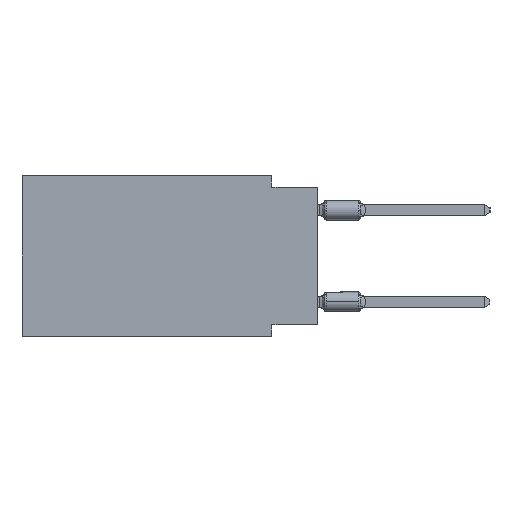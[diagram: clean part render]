
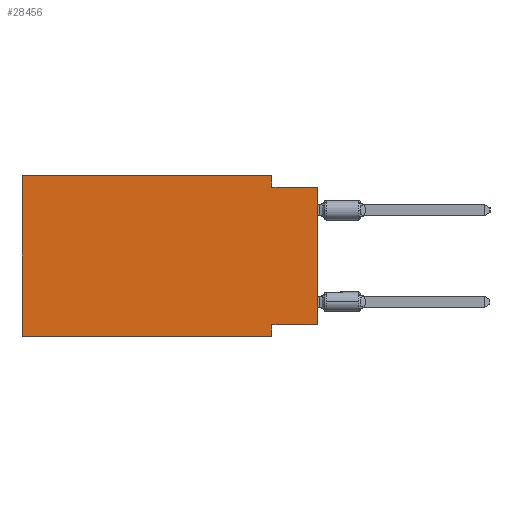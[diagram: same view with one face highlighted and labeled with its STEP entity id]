
A CAD part, left-side view. The second image highlights one B-rep face of the part: STEP entity #28456.
In plain terms, the highlighted planar face has unit normal (-1, 0, 0).
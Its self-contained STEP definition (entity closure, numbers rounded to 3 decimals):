
#618 = EDGE_CURVE ( 'NONE', #53708, #17051, #42193, .T. ) ;
#4104 = CARTESIAN_POINT ( 'NONE',  ( 0., 16.383, 0. ) ) ;
#4220 = ORIENTED_EDGE ( 'NONE', *, *, #20151, .F. ) ;
#5010 = VECTOR ( 'NONE', #34080, 1000. ) ;
#5094 = PLANE ( 'NONE',  #58560 ) ;
#6887 = CARTESIAN_POINT ( 'NONE',  ( 0., 0., -0.635 ) ) ;
#7912 = VECTOR ( 'NONE', #18733, 1000. ) ;
#11517 = CARTESIAN_POINT ( 'NONE',  ( 0., 0., 0. ) ) ;
#12225 = LINE ( 'NONE', #44247, #46390 ) ;
#13264 = EDGE_CURVE ( 'NONE', #17971, #17051, #45311, .T. ) ;
#13983 = ORIENTED_EDGE ( 'NONE', *, *, #56285, .F. ) ;
#17051 = VERTEX_POINT ( 'NONE', #6887 ) ;
#17971 = VERTEX_POINT ( 'NONE', #45802 ) ;
#18733 = DIRECTION ( 'NONE',  ( 0., -1., 0. ) ) ;
#19631 = VECTOR ( 'NONE', #56861, 1000. ) ;
#19765 = CARTESIAN_POINT ( 'NONE',  ( 0., 16.383, 0. ) ) ;
#20151 = EDGE_CURVE ( 'NONE', #31543, #17971, #60841, .T. ) ;
#21318 = EDGE_CURVE ( 'NONE', #53708, #58305, #46108, .T. ) ;
#24702 = ORIENTED_EDGE ( 'NONE', *, *, #34564, .T. ) ;
#24918 = CARTESIAN_POINT ( 'NONE',  ( 0., 0., -8.255 ) ) ;
#25700 = EDGE_CURVE ( 'NONE', #61450, #31543, #46005, .T. ) ;
#26708 = ORIENTED_EDGE ( 'NONE', *, *, #21318, .F. ) ;
#28456 = ADVANCED_FACE ( 'NONE', ( #51433 ), #5094, .F. ) ;
#30171 = DIRECTION ( 'NONE',  ( 0., 0., -1. ) ) ;
#31422 = CARTESIAN_POINT ( 'NONE',  ( 0., 2.54, 0. ) ) ;
#31543 = VERTEX_POINT ( 'NONE', #31422 ) ;
#33011 = DIRECTION ( 'NONE',  ( 0., 0., -1. ) ) ;
#33421 = ORIENTED_EDGE ( 'NONE', *, *, #25700, .F. ) ;
#33478 = CARTESIAN_POINT ( 'NONE',  ( 0., 16.383, 0. ) ) ;
#34080 = DIRECTION ( 'NONE',  ( 0., -1., 0. ) ) ;
#34564 = EDGE_CURVE ( 'NONE', #39815, #61401, #39172, .T. ) ;
#35756 = DIRECTION ( 'NONE',  ( 1., 0., 0. ) ) ;
#36201 = DIRECTION ( 'NONE',  ( 0., 1., 0. ) ) ;
#36923 = VECTOR ( 'NONE', #36201, 1000. ) ;
#38734 = ORIENTED_EDGE ( 'NONE', *, *, #618, .T. ) ;
#39172 = LINE ( 'NONE', #59972, #5010 ) ;
#39815 = VERTEX_POINT ( 'NONE', #63737 ) ;
#39867 = CARTESIAN_POINT ( 'NONE',  ( 0., 2.54, -8.89 ) ) ;
#41205 = DIRECTION ( 'NONE',  ( 0., 0., -1. ) ) ;
#42193 = LINE ( 'NONE', #11517, #19631 ) ;
#42225 = VECTOR ( 'NONE', #30171, 1000. ) ;
#42566 = ORIENTED_EDGE ( 'NONE', *, *, #13264, .F. ) ;
#44247 = CARTESIAN_POINT ( 'NONE',  ( 0., 2.54, -8.89 ) ) ;
#44613 = VECTOR ( 'NONE', #49166, 1000. ) ;
#44979 = DIRECTION ( 'NONE',  ( 0., -1., 0. ) ) ;
#45311 = LINE ( 'NONE', #45990, #7912 ) ;
#45802 = CARTESIAN_POINT ( 'NONE',  ( 0., 2.54, -0.635 ) ) ;
#45990 = CARTESIAN_POINT ( 'NONE',  ( 0., 0., -0.635 ) ) ;
#46005 = LINE ( 'NONE', #4104, #64182 ) ;
#46108 = LINE ( 'NONE', #66872, #36923 ) ;
#46390 = VECTOR ( 'NONE', #33011, 1000. ) ;
#49166 = DIRECTION ( 'NONE',  ( 0., 0., 1. ) ) ;
#50500 = LINE ( 'NONE', #33478, #44613 ) ;
#51433 = FACE_OUTER_BOUND ( 'NONE', #61198, .T. ) ;
#53708 = VERTEX_POINT ( 'NONE', #24918 ) ;
#55894 = CARTESIAN_POINT ( 'NONE',  ( 0., 16.383, 0. ) ) ;
#56285 = EDGE_CURVE ( 'NONE', #58305, #61401, #12225, .T. ) ;
#56861 = DIRECTION ( 'NONE',  ( 0., 0., 1. ) ) ;
#58305 = VERTEX_POINT ( 'NONE', #63749 ) ;
#58560 = AXIS2_PLACEMENT_3D ( 'NONE', #19765, #35756, #41205 ) ;
#59834 = CARTESIAN_POINT ( 'NONE',  ( 0., 2.54, 0. ) ) ;
#59972 = CARTESIAN_POINT ( 'NONE',  ( 0., 16.383, -8.89 ) ) ;
#60841 = LINE ( 'NONE', #59834, #42225 ) ;
#61198 = EDGE_LOOP ( 'NONE', ( #38734, #42566, #4220, #33421, #64127, #24702, #13983, #26708 ) ) ;
#61401 = VERTEX_POINT ( 'NONE', #39867 ) ;
#61450 = VERTEX_POINT ( 'NONE', #55894 ) ;
#62789 = EDGE_CURVE ( 'NONE', #39815, #61450, #50500, .T. ) ;
#63737 = CARTESIAN_POINT ( 'NONE',  ( 0., 16.383, -8.89 ) ) ;
#63749 = CARTESIAN_POINT ( 'NONE',  ( 0., 2.54, -8.255 ) ) ;
#64127 = ORIENTED_EDGE ( 'NONE', *, *, #62789, .F. ) ;
#64182 = VECTOR ( 'NONE', #44979, 1000. ) ;
#66872 = CARTESIAN_POINT ( 'NONE',  ( 0., 0., -8.255 ) ) ;
